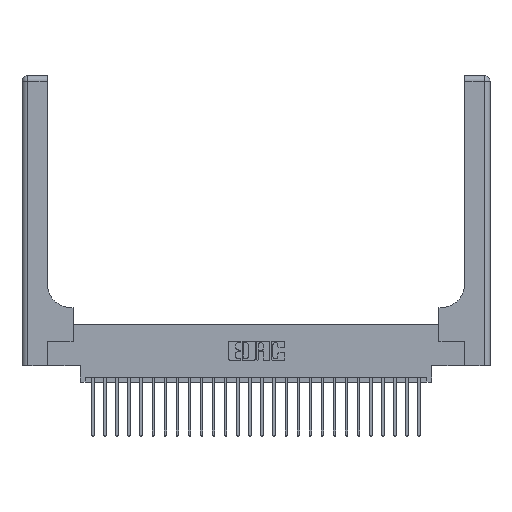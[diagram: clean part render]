
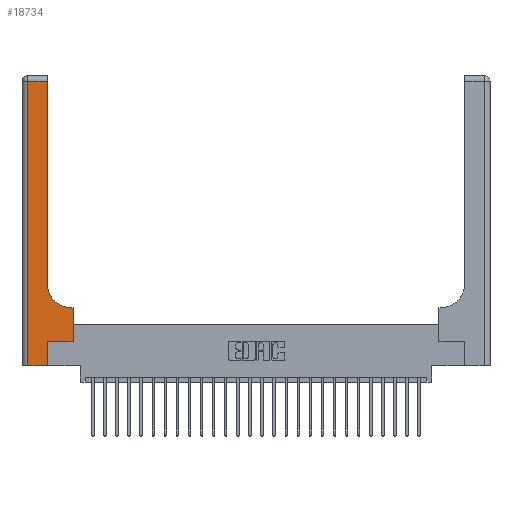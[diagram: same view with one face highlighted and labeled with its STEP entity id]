
A CAD part, top view. The second image highlights one B-rep face of the part: STEP entity #18734.
In plain terms, the highlighted planar face has unit normal (0, 0, 1).
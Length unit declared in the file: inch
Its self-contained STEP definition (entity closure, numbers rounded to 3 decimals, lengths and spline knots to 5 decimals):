
#443 = DIRECTION ( 'NONE',  ( -1., 0., 0. ) ) ;
#629 = ORIENTED_EDGE ( 'NONE', *, *, #9002, .T. ) ;
#1010 = LINE ( 'NONE', #22085, #22001 ) ;
#1640 = VERTEX_POINT ( 'NONE', #22964 ) ;
#1685 = EDGE_CURVE ( 'NONE', #24299, #13999, #16936, .T. ) ;
#2056 = CARTESIAN_POINT ( 'NONE',  ( 0.265, 0., 0.37 ) ) ;
#3379 = AXIS2_PLACEMENT_3D ( 'NONE', #10134, #23853, #12129 ) ;
#3426 = CARTESIAN_POINT ( 'NONE',  ( 0.265, 0.25, 0.37 ) ) ;
#4167 = VECTOR ( 'NONE', #13539, 39.37008 ) ;
#4406 = EDGE_CURVE ( 'NONE', #22844, #25504, #24498, .T. ) ;
#4562 = CARTESIAN_POINT ( 'NONE',  ( 0.528, 0.25, 0.37 ) ) ;
#4857 = EDGE_CURVE ( 'NONE', #1640, #22844, #14091, .T. ) ;
#5021 = DIRECTION ( 'NONE',  ( 0., 1., 0. ) ) ;
#5699 = CARTESIAN_POINT ( 'NONE',  ( 0.26, 2.94, 0.37 ) ) ;
#5787 = ORIENTED_EDGE ( 'NONE', *, *, #9984, .T. ) ;
#6024 = CARTESIAN_POINT ( 'NONE',  ( 0., 0., 0.37 ) ) ;
#6308 = CARTESIAN_POINT ( 'NONE',  ( 0.26, 0.85, 0.37 ) ) ;
#6557 = DIRECTION ( 'NONE',  ( 0., 1., 0. ) ) ;
#6713 = AXIS2_PLACEMENT_3D ( 'NONE', #8348, #12334, #443 ) ;
#7009 = CARTESIAN_POINT ( 'NONE',  ( 0.26, 3., 0.37 ) ) ;
#7580 = DIRECTION ( 'NONE',  ( -1., 0., 0. ) ) ;
#7642 = CARTESIAN_POINT ( 'NONE',  ( 0.528, 0.25, 0.37 ) ) ;
#8087 = VECTOR ( 'NONE', #7580, 39.37008 ) ;
#8348 = CARTESIAN_POINT ( 'NONE',  ( 0., 3., 0.37 ) ) ;
#8757 = LINE ( 'NONE', #4562, #23791 ) ;
#8938 = EDGE_LOOP ( 'NONE', ( #14133, #5787, #16799, #24582, #10620, #10141, #629, #23265, #15916 ) ) ;
#9002 = EDGE_CURVE ( 'NONE', #13999, #13283, #8757, .T. ) ;
#9984 = EDGE_CURVE ( 'NONE', #19742, #1640, #18570, .T. ) ;
#10090 = VECTOR ( 'NONE', #21770, 39.37008 ) ;
#10134 = CARTESIAN_POINT ( 'NONE',  ( 0.51, 0.85, 0.37 ) ) ;
#10141 = ORIENTED_EDGE ( 'NONE', *, *, #1685, .T. ) ;
#10620 = ORIENTED_EDGE ( 'NONE', *, *, #16010, .T. ) ;
#10630 = CARTESIAN_POINT ( 'NONE',  ( 0.51, 0.6, 0.37 ) ) ;
#11588 = CARTESIAN_POINT ( 'NONE',  ( 0., 2.94, 0.37 ) ) ;
#12129 = DIRECTION ( 'NONE',  ( 1., 0., 0. ) ) ;
#12334 = DIRECTION ( 'NONE',  ( 0., 0., -1. ) ) ;
#13283 = VERTEX_POINT ( 'NONE', #20939 ) ;
#13539 = DIRECTION ( 'NONE',  ( 0., -1., 0. ) ) ;
#13921 = FACE_OUTER_BOUND ( 'NONE', #8938, .T. ) ;
#13938 = DIRECTION ( 'NONE',  ( 0., 1., 0. ) ) ;
#13999 = VERTEX_POINT ( 'NONE', #7642 ) ;
#14069 = CIRCLE ( 'NONE', #3379, 0.25 ) ;
#14091 = LINE ( 'NONE', #25233, #4167 ) ;
#14133 = ORIENTED_EDGE ( 'NONE', *, *, #17507, .T. ) ;
#14168 = CARTESIAN_POINT ( 'NONE',  ( 0.265, 0.25, 0.37 ) ) ;
#14233 = EDGE_CURVE ( 'NONE', #13283, #20078, #1010, .T. ) ;
#14833 = EDGE_CURVE ( 'NONE', #20078, #17948, #14069, .T. ) ;
#14981 = VECTOR ( 'NONE', #13938, 39.37008 ) ;
#15916 = ORIENTED_EDGE ( 'NONE', *, *, #14833, .T. ) ;
#16010 = EDGE_CURVE ( 'NONE', #25504, #24299, #25352, .T. ) ;
#16799 = ORIENTED_EDGE ( 'NONE', *, *, #4857, .T. ) ;
#16936 = LINE ( 'NONE', #3426, #22116 ) ;
#17507 = EDGE_CURVE ( 'NONE', #17948, #19742, #18887, .T. ) ;
#17948 = VERTEX_POINT ( 'NONE', #6308 ) ;
#18570 = LINE ( 'NONE', #11588, #8087 ) ;
#18734 = ADVANCED_FACE ( 'NONE', ( #13921 ), #24052, .F. ) ;
#18887 = LINE ( 'NONE', #7009, #23445 ) ;
#19224 = DIRECTION ( 'NONE',  ( 1., 0., 0. ) ) ;
#19242 = CARTESIAN_POINT ( 'NONE',  ( 0.265, 0., 0.37 ) ) ;
#19742 = VERTEX_POINT ( 'NONE', #5699 ) ;
#20078 = VERTEX_POINT ( 'NONE', #10630 ) ;
#20939 = CARTESIAN_POINT ( 'NONE',  ( 0.528, 0.6, 0.37 ) ) ;
#21770 = DIRECTION ( 'NONE',  ( 1., 0., 0. ) ) ;
#22001 = VECTOR ( 'NONE', #24042, 39.37008 ) ;
#22085 = CARTESIAN_POINT ( 'NONE',  ( 0.26, 0.6, 0.37 ) ) ;
#22116 = VECTOR ( 'NONE', #19224, 39.37008 ) ;
#22844 = VERTEX_POINT ( 'NONE', #25409 ) ;
#22964 = CARTESIAN_POINT ( 'NONE',  ( 0.06, 2.94, 0.37 ) ) ;
#23265 = ORIENTED_EDGE ( 'NONE', *, *, #14233, .T. ) ;
#23445 = VECTOR ( 'NONE', #5021, 39.37008 ) ;
#23791 = VECTOR ( 'NONE', #6557, 39.37008 ) ;
#23853 = DIRECTION ( 'NONE',  ( 0., 0., -1. ) ) ;
#24042 = DIRECTION ( 'NONE',  ( -1., 0., 0. ) ) ;
#24052 = PLANE ( 'NONE',  #6713 ) ;
#24299 = VERTEX_POINT ( 'NONE', #14168 ) ;
#24498 = LINE ( 'NONE', #6024, #10090 ) ;
#24582 = ORIENTED_EDGE ( 'NONE', *, *, #4406, .T. ) ;
#25233 = CARTESIAN_POINT ( 'NONE',  ( 0.06, 3., 0.37 ) ) ;
#25352 = LINE ( 'NONE', #2056, #14981 ) ;
#25409 = CARTESIAN_POINT ( 'NONE',  ( 0.06, 0., 0.37 ) ) ;
#25504 = VERTEX_POINT ( 'NONE', #19242 ) ;
